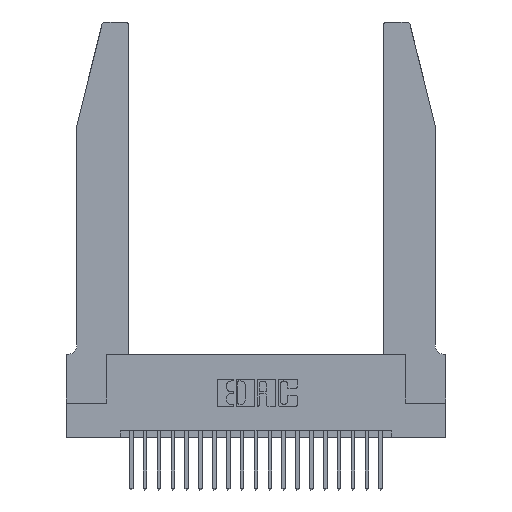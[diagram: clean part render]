
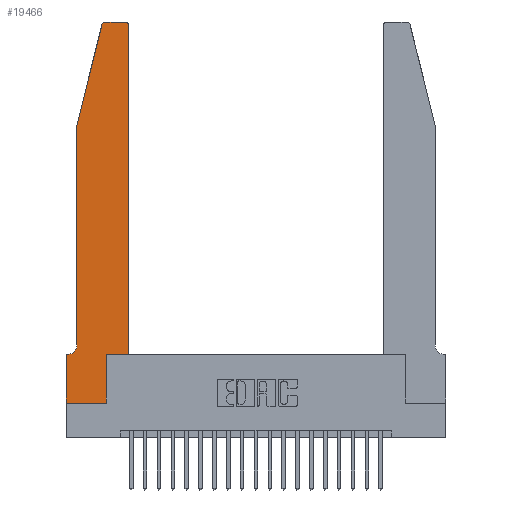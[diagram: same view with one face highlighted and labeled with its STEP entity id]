
A CAD part, top view. The second image highlights one B-rep face of the part: STEP entity #19466.
In plain terms, the highlighted planar face has unit normal (0, 0, 1).
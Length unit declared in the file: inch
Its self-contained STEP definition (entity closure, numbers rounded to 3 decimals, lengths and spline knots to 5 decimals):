
#71 = CARTESIAN_POINT ( 'NONE',  ( 0.0755, 2., 0.37 ) ) ;
#93 = VECTOR ( 'NONE', #11102, 39.37008 ) ;
#139 = VECTOR ( 'NONE', #21951, 39.37008 ) ;
#609 = EDGE_CURVE ( 'NONE', #7422, #14229, #17303, .T. ) ;
#770 = AXIS2_PLACEMENT_3D ( 'NONE', #17705, #7128, #3743 ) ;
#810 = CARTESIAN_POINT ( 'NONE',  ( 0.0755, 0.42, 0.37 ) ) ;
#930 = ORIENTED_EDGE ( 'NONE', *, *, #17563, .T. ) ;
#944 = ORIENTED_EDGE ( 'NONE', *, *, #13877, .T. ) ;
#988 = CIRCLE ( 'NONE', #770, 0.03 ) ;
#1101 = CARTESIAN_POINT ( 'NONE',  ( 0.4205, 2.72, 0.37 ) ) ;
#1182 = EDGE_CURVE ( 'NONE', #5298, #21280, #16484, .T. ) ;
#1519 = CARTESIAN_POINT ( 'NONE',  ( 0.0755, 2., 0.37 ) ) ;
#1626 = LINE ( 'NONE', #9758, #19824 ) ;
#2120 = DIRECTION ( 'NONE',  ( 1., 0., 0. ) ) ;
#2233 = EDGE_CURVE ( 'NONE', #21280, #4912, #20312, .T. ) ;
#3654 = LINE ( 'NONE', #7395, #93 ) ;
#3675 = VERTEX_POINT ( 'NONE', #13629 ) ;
#3704 = DIRECTION ( 'NONE',  ( -1., 0., 0. ) ) ;
#3743 = DIRECTION ( 'NONE',  ( 1., 0., 0. ) ) ;
#3824 = EDGE_CURVE ( 'NONE', #8162, #12615, #4836, .T. ) ;
#3887 = EDGE_LOOP ( 'NONE', ( #16318, #930, #944, #14257, #9973, #19439, #21507, #17520, #9059, #4277, #6344, #19986 ) ) ;
#4176 = CARTESIAN_POINT ( 'NONE',  ( 0.0055, 0.35, 0.37 ) ) ;
#4199 = CARTESIAN_POINT ( 'NONE',  ( 0.2605, 2.75, 0.37 ) ) ;
#4242 = LINE ( 'NONE', #7492, #13598 ) ;
#4277 = ORIENTED_EDGE ( 'NONE', *, *, #609, .T. ) ;
#4408 = LINE ( 'NONE', #15274, #5524 ) ;
#4750 = CARTESIAN_POINT ( 'NONE',  ( 0.284, 2.75, 0.37 ) ) ;
#4806 = DIRECTION ( 'NONE',  ( 1., 0., 0. ) ) ;
#4836 = LINE ( 'NONE', #11146, #139 ) ;
#4912 = VERTEX_POINT ( 'NONE', #4176 ) ;
#5112 = EDGE_CURVE ( 'NONE', #3675, #8162, #3654, .T. ) ;
#5298 = VERTEX_POINT ( 'NONE', #1519 ) ;
#5524 = VECTOR ( 'NONE', #15046, 39.37008 ) ;
#6344 = ORIENTED_EDGE ( 'NONE', *, *, #18348, .T. ) ;
#7128 = DIRECTION ( 'NONE',  ( 0., 0., 1. ) ) ;
#7358 = PLANE ( 'NONE',  #20985 ) ;
#7376 = LINE ( 'NONE', #4199, #20844 ) ;
#7395 = CARTESIAN_POINT ( 'NONE',  ( 0., 0., 0.37 ) ) ;
#7422 = VERTEX_POINT ( 'NONE', #13955 ) ;
#7492 = CARTESIAN_POINT ( 'NONE',  ( 0.4505, 0.35, 0.37 ) ) ;
#8067 = VERTEX_POINT ( 'NONE', #12790 ) ;
#8162 = VERTEX_POINT ( 'NONE', #11410 ) ;
#8439 = CARTESIAN_POINT ( 'NONE',  ( 0.4505, 0.35, 0.37 ) ) ;
#9059 = ORIENTED_EDGE ( 'NONE', *, *, #12436, .T. ) ;
#9147 = CARTESIAN_POINT ( 'NONE',  ( 0.4505, 0.35, 0.37 ) ) ;
#9758 = CARTESIAN_POINT ( 'NONE',  ( 0.0755, 2., 0.37 ) ) ;
#9973 = ORIENTED_EDGE ( 'NONE', *, *, #2233, .T. ) ;
#10842 = CARTESIAN_POINT ( 'NONE',  ( 0., 0.35, 0.37 ) ) ;
#11102 = DIRECTION ( 'NONE',  ( 0., -1., 0. ) ) ;
#11146 = CARTESIAN_POINT ( 'NONE',  ( 0., 0., 0.37 ) ) ;
#11355 = DIRECTION ( 'NONE',  ( 0., 1., 0. ) ) ;
#11366 = VERTEX_POINT ( 'NONE', #4750 ) ;
#11410 = CARTESIAN_POINT ( 'NONE',  ( 0., 0., 0.37 ) ) ;
#11861 = EDGE_CURVE ( 'NONE', #17217, #8067, #12705, .T. ) ;
#12436 = EDGE_CURVE ( 'NONE', #12615, #7422, #4408, .T. ) ;
#12615 = VERTEX_POINT ( 'NONE', #15587 ) ;
#12705 = CIRCLE ( 'NONE', #22060, 0.03 ) ;
#12790 = CARTESIAN_POINT ( 'NONE',  ( 0.4205, 2.75, 0.37 ) ) ;
#13129 = VECTOR ( 'NONE', #19567, 39.37008 ) ;
#13209 = DIRECTION ( 'NONE',  ( -1., 0., 0. ) ) ;
#13236 = DIRECTION ( 'NONE',  ( -0.239, -0.971, 0. ) ) ;
#13381 = LINE ( 'NONE', #20675, #20008 ) ;
#13598 = VECTOR ( 'NONE', #11355, 39.37008 ) ;
#13629 = CARTESIAN_POINT ( 'NONE',  ( 0., 0.35, 0.37 ) ) ;
#13770 = DIRECTION ( 'NONE',  ( 1., 0., 0. ) ) ;
#13877 = EDGE_CURVE ( 'NONE', #19319, #5298, #1626, .T. ) ;
#13955 = CARTESIAN_POINT ( 'NONE',  ( 0.2865, 0.35, 0.37 ) ) ;
#14229 = VERTEX_POINT ( 'NONE', #9147 ) ;
#14257 = ORIENTED_EDGE ( 'NONE', *, *, #1182, .T. ) ;
#14505 = EDGE_CURVE ( 'NONE', #8067, #11366, #7376, .T. ) ;
#15046 = DIRECTION ( 'NONE',  ( 0., 1., 0. ) ) ;
#15274 = CARTESIAN_POINT ( 'NONE',  ( 0.2865, 0.35, 0.37 ) ) ;
#15587 = CARTESIAN_POINT ( 'NONE',  ( 0.2865, 0., 0.37 ) ) ;
#15773 = AXIS2_PLACEMENT_3D ( 'NONE', #16224, #17823, #3704 ) ;
#16224 = CARTESIAN_POINT ( 'NONE',  ( 0.0055, 0.42, 0.37 ) ) ;
#16256 = DIRECTION ( 'NONE',  ( 0., 0., 1. ) ) ;
#16318 = ORIENTED_EDGE ( 'NONE', *, *, #14505, .T. ) ;
#16484 = LINE ( 'NONE', #71, #13129 ) ;
#16645 = CARTESIAN_POINT ( 'NONE',  ( 0.4505, 2.72, 0.37 ) ) ;
#17217 = VERTEX_POINT ( 'NONE', #16645 ) ;
#17238 = DIRECTION ( 'NONE',  ( -1., 0., 0. ) ) ;
#17277 = DIRECTION ( 'NONE',  ( 0., 0., 1. ) ) ;
#17303 = LINE ( 'NONE', #8439, #21424 ) ;
#17357 = EDGE_CURVE ( 'NONE', #4912, #3675, #13381, .T. ) ;
#17520 = ORIENTED_EDGE ( 'NONE', *, *, #3824, .T. ) ;
#17563 = EDGE_CURVE ( 'NONE', #11366, #19319, #988, .T. ) ;
#17705 = CARTESIAN_POINT ( 'NONE',  ( 0.284, 2.72, 0.37 ) ) ;
#17823 = DIRECTION ( 'NONE',  ( 0., 0., -1. ) ) ;
#18348 = EDGE_CURVE ( 'NONE', #14229, #17217, #4242, .T. ) ;
#19219 = CARTESIAN_POINT ( 'NONE',  ( 0.25487, 2.72718, 0.37 ) ) ;
#19319 = VERTEX_POINT ( 'NONE', #19219 ) ;
#19439 = ORIENTED_EDGE ( 'NONE', *, *, #17357, .T. ) ;
#19466 = ADVANCED_FACE ( 'NONE', ( #20986 ), #7358, .T. ) ;
#19567 = DIRECTION ( 'NONE',  ( 0., -1., 0. ) ) ;
#19824 = VECTOR ( 'NONE', #13236, 39.37008 ) ;
#19986 = ORIENTED_EDGE ( 'NONE', *, *, #11861, .T. ) ;
#20008 = VECTOR ( 'NONE', #17238, 39.37008 ) ;
#20312 = CIRCLE ( 'NONE', #15773, 0.07 ) ;
#20675 = CARTESIAN_POINT ( 'NONE',  ( 0.0755, 0.35, 0.37 ) ) ;
#20844 = VECTOR ( 'NONE', #13209, 39.37008 ) ;
#20985 = AXIS2_PLACEMENT_3D ( 'NONE', #10842, #16256, #2120 ) ;
#20986 = FACE_OUTER_BOUND ( 'NONE', #3887, .T. ) ;
#21280 = VERTEX_POINT ( 'NONE', #810 ) ;
#21424 = VECTOR ( 'NONE', #13770, 39.37008 ) ;
#21507 = ORIENTED_EDGE ( 'NONE', *, *, #5112, .T. ) ;
#21951 = DIRECTION ( 'NONE',  ( 1., 0., 0. ) ) ;
#22060 = AXIS2_PLACEMENT_3D ( 'NONE', #1101, #17277, #4806 ) ;
